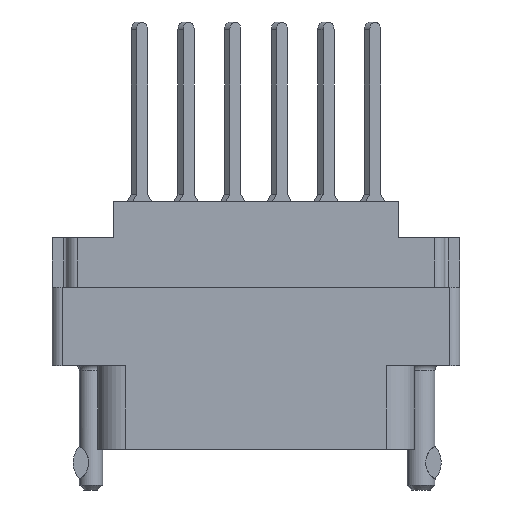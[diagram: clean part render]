
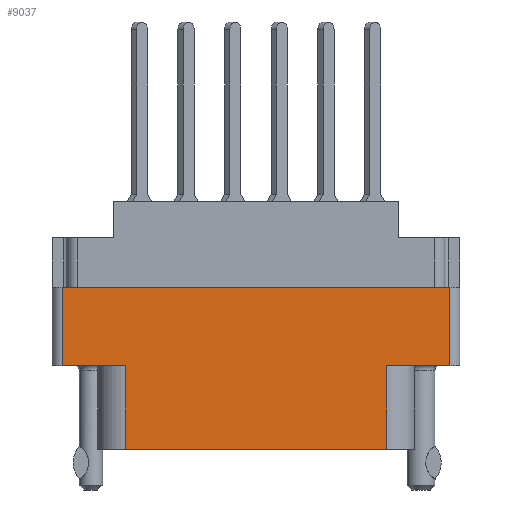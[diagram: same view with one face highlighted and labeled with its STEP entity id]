
A CAD part, front view. The second image highlights one B-rep face of the part: STEP entity #9037.
In plain terms, the highlighted planar face has unit normal (0, -1, 0).
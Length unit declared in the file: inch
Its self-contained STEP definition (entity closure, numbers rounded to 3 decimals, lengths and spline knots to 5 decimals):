
#92 = LINE ( 'NONE', #5725, #27621 ) ;
#470 = VECTOR ( 'NONE', #32910, 39.37008 ) ;
#600 = LINE ( 'NONE', #28063, #1036 ) ;
#705 = DIRECTION ( 'NONE',  ( 0., 0., -1. ) ) ;
#1036 = VECTOR ( 'NONE', #23007, 39.37008 ) ;
#1482 = ORIENTED_EDGE ( 'NONE', *, *, #24289, .F. ) ;
#1748 = CARTESIAN_POINT ( 'NONE',  ( 0., -0.343, -0.529 ) ) ;
#2550 = ORIENTED_EDGE ( 'NONE', *, *, #25725, .T. ) ;
#2562 = EDGE_CURVE ( 'NONE', #22207, #31959, #32128, .T. ) ;
#2853 = LINE ( 'NONE', #13356, #30372 ) ;
#3247 = AXIS2_PLACEMENT_3D ( 'NONE', #4592, #12391, #30464 ) ;
#4592 = CARTESIAN_POINT ( 'NONE',  ( -0.624, -0.343, -0.798 ) ) ;
#4663 = DIRECTION ( 'NONE',  ( 0., 0., 1. ) ) ;
#4734 = ORIENTED_EDGE ( 'NONE', *, *, #24018, .F. ) ;
#4975 = CARTESIAN_POINT ( 'NONE',  ( -0.42, -0.343, -0.529 ) ) ;
#5725 = CARTESIAN_POINT ( 'NONE',  ( 0.42, -0.343, -0.529 ) ) ;
#6021 = VERTEX_POINT ( 'NONE', #7374 ) ;
#6878 = ORIENTED_EDGE ( 'NONE', *, *, #2562, .F. ) ;
#7374 = CARTESIAN_POINT ( 'NONE',  ( 0.42, -0.343, -0.798 ) ) ;
#8545 = CARTESIAN_POINT ( 'NONE',  ( -0.624, -0.343, -0.277 ) ) ;
#9037 = ADVANCED_FACE ( 'NONE', ( #33136 ), #20045, .T. ) ;
#9105 = VECTOR ( 'NONE', #12874, 39.37008 ) ;
#9733 = CARTESIAN_POINT ( 'NONE',  ( -0.624, -0.343, -0.798 ) ) ;
#10633 = LINE ( 'NONE', #19519, #21124 ) ;
#11014 = EDGE_CURVE ( 'NONE', #27442, #14377, #21232, .T. ) ;
#11972 = DIRECTION ( 'NONE',  ( 1., 0., 0. ) ) ;
#12337 = CARTESIAN_POINT ( 'NONE',  ( 0.624, -0.343, -0.798 ) ) ;
#12391 = DIRECTION ( 'NONE',  ( 0., -1., 0. ) ) ;
#12456 = CARTESIAN_POINT ( 'NONE',  ( -0.42, -0.343, -0.529 ) ) ;
#12874 = DIRECTION ( 'NONE',  ( 0., 0., -1. ) ) ;
#13244 = ORIENTED_EDGE ( 'NONE', *, *, #27803, .T. ) ;
#13356 = CARTESIAN_POINT ( 'NONE',  ( -0.656, -0.343, -0.277 ) ) ;
#14377 = VERTEX_POINT ( 'NONE', #20865 ) ;
#15741 = ORIENTED_EDGE ( 'NONE', *, *, #11014, .T. ) ;
#19519 = CARTESIAN_POINT ( 'NONE',  ( 0., -0.343, -0.529 ) ) ;
#19949 = VECTOR ( 'NONE', #4663, 39.37008 ) ;
#20045 = PLANE ( 'NONE',  #3247 ) ;
#20808 = CARTESIAN_POINT ( 'NONE',  ( 0.624, -0.343, -0.529 ) ) ;
#20865 = CARTESIAN_POINT ( 'NONE',  ( -0.42, -0.343, -0.798 ) ) ;
#21099 = VERTEX_POINT ( 'NONE', #8545 ) ;
#21124 = VECTOR ( 'NONE', #11972, 39.37008 ) ;
#21232 = LINE ( 'NONE', #4975, #9105 ) ;
#21516 = VERTEX_POINT ( 'NONE', #29587 ) ;
#22072 = EDGE_CURVE ( 'NONE', #31959, #6021, #92, .T. ) ;
#22207 = VERTEX_POINT ( 'NONE', #20808 ) ;
#22329 = DIRECTION ( 'NONE',  ( -1., 0., 0. ) ) ;
#22330 = ORIENTED_EDGE ( 'NONE', *, *, #27961, .T. ) ;
#23007 = DIRECTION ( 'NONE',  ( 1., 0., 0. ) ) ;
#24018 = EDGE_CURVE ( 'NONE', #21099, #21516, #2853, .T. ) ;
#24289 = EDGE_CURVE ( 'NONE', #32270, #21099, #28484, .T. ) ;
#25594 = EDGE_LOOP ( 'NONE', ( #15741, #2550, #29841, #6878, #22330, #4734, #1482, #13244 ) ) ;
#25725 = EDGE_CURVE ( 'NONE', #14377, #6021, #600, .T. ) ;
#27442 = VERTEX_POINT ( 'NONE', #12456 ) ;
#27621 = VECTOR ( 'NONE', #705, 39.37008 ) ;
#27803 = EDGE_CURVE ( 'NONE', #32270, #27442, #10633, .T. ) ;
#27961 = EDGE_CURVE ( 'NONE', #22207, #21516, #32903, .T. ) ;
#28063 = CARTESIAN_POINT ( 'NONE',  ( -0.624, -0.343, -0.798 ) ) ;
#28484 = LINE ( 'NONE', #9733, #19949 ) ;
#28811 = CARTESIAN_POINT ( 'NONE',  ( 0.42, -0.343, -0.529 ) ) ;
#29587 = CARTESIAN_POINT ( 'NONE',  ( 0.624, -0.343, -0.277 ) ) ;
#29841 = ORIENTED_EDGE ( 'NONE', *, *, #22072, .F. ) ;
#30372 = VECTOR ( 'NONE', #31325, 39.37008 ) ;
#30464 = DIRECTION ( 'NONE',  ( 0., 0., -1. ) ) ;
#31325 = DIRECTION ( 'NONE',  ( 1., 0., 0. ) ) ;
#31689 = VECTOR ( 'NONE', #22329, 39.37008 ) ;
#31959 = VERTEX_POINT ( 'NONE', #28811 ) ;
#32128 = LINE ( 'NONE', #1748, #31689 ) ;
#32191 = CARTESIAN_POINT ( 'NONE',  ( -0.624, -0.343, -0.529 ) ) ;
#32270 = VERTEX_POINT ( 'NONE', #32191 ) ;
#32903 = LINE ( 'NONE', #12337, #470 ) ;
#32910 = DIRECTION ( 'NONE',  ( 0., 0., 1. ) ) ;
#33136 = FACE_OUTER_BOUND ( 'NONE', #25594, .T. ) ;
